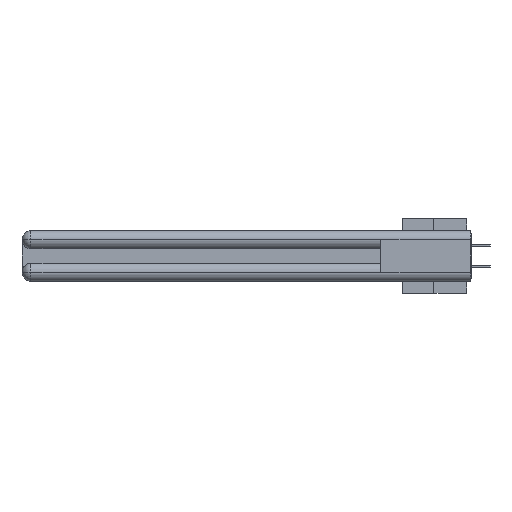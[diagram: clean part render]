
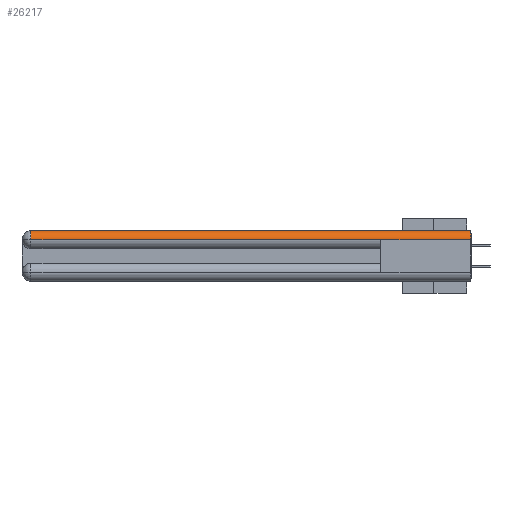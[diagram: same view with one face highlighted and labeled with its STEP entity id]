
A CAD part, left-side view. The second image highlights one B-rep face of the part: STEP entity #26217.
In plain terms, the highlighted cylindrical face has radius 1.562 mm (diameter 3.124 mm), a partial arc.
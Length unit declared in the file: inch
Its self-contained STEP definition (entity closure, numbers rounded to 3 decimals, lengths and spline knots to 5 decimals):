
#1424 = CARTESIAN_POINT ( 'NONE',  ( 0., 0., -0.0615 ) ) ;
#1854 = VERTEX_POINT ( 'NONE', #1424 ) ;
#3179 = VERTEX_POINT ( 'NONE', #27370 ) ;
#4358 = DIRECTION ( 'NONE',  ( 0., -1., 0. ) ) ;
#4647 = VECTOR ( 'NONE', #32517, 39.37008 ) ;
#5526 = ORIENTED_EDGE ( 'NONE', *, *, #14792, .F. ) ;
#6897 = VERTEX_POINT ( 'NONE', #30678 ) ;
#6945 = VERTEX_POINT ( 'NONE', #16879 ) ;
#8374 = EDGE_CURVE ( 'NONE', #6897, #30073, #10046, .T. ) ;
#8492 = EDGE_LOOP ( 'NONE', ( #33950, #23295, #24960, #5526, #19965 ) ) ;
#8724 = LINE ( 'NONE', #32281, #4647 ) ;
#10006 = CARTESIAN_POINT ( 'NONE',  ( 0., 3., -0.0615 ) ) ;
#10046 = CIRCLE ( 'NONE', #24034, 0.0615 ) ;
#11680 = DIRECTION ( 'NONE',  ( 0., 0., 1. ) ) ;
#11841 = VECTOR ( 'NONE', #4358, 39.37008 ) ;
#11908 = CARTESIAN_POINT ( 'NONE',  ( 0., 2.94, -0.0615 ) ) ;
#12241 = LINE ( 'NONE', #20618, #34445 ) ;
#13191 = CARTESIAN_POINT ( 'NONE',  ( 0.0615, 2.94, -0.0615 ) ) ;
#14202 = DIRECTION ( 'NONE',  ( 1., 0., 0. ) ) ;
#14792 = EDGE_CURVE ( 'NONE', #1854, #3179, #12241, .T. ) ;
#15182 = DIRECTION ( 'NONE',  ( 0., 1., 0. ) ) ;
#16879 = CARTESIAN_POINT ( 'NONE',  ( 0.0615, 0., 0. ) ) ;
#17101 = DIRECTION ( 'NONE',  ( 0., -1., 0. ) ) ;
#18936 = CARTESIAN_POINT ( 'NONE',  ( 0.0615, 0., -0.0615 ) ) ;
#19277 = AXIS2_PLACEMENT_3D ( 'NONE', #31559, #17101, #14202 ) ;
#19965 = ORIENTED_EDGE ( 'NONE', *, *, #31955, .F. ) ;
#20372 = LINE ( 'NONE', #10006, #11841 ) ;
#20618 = CARTESIAN_POINT ( 'NONE',  ( 0., 3., -0.0615 ) ) ;
#23295 = ORIENTED_EDGE ( 'NONE', *, *, #8374, .T. ) ;
#23879 = EDGE_CURVE ( 'NONE', #6897, #6945, #8724, .T. ) ;
#24034 = AXIS2_PLACEMENT_3D ( 'NONE', #13191, #36397, #36026 ) ;
#24771 = DIRECTION ( 'NONE',  ( 0., 1., 0. ) ) ;
#24960 = ORIENTED_EDGE ( 'NONE', *, *, #32616, .T. ) ;
#26056 = FACE_OUTER_BOUND ( 'NONE', #8492, .T. ) ;
#26217 = ADVANCED_FACE ( 'NONE', ( #26056 ), #32856, .T. ) ;
#27370 = CARTESIAN_POINT ( 'NONE',  ( 0., 0.6, -0.0615 ) ) ;
#30073 = VERTEX_POINT ( 'NONE', #11908 ) ;
#30678 = CARTESIAN_POINT ( 'NONE',  ( 0.0615, 2.94, 0. ) ) ;
#31274 = AXIS2_PLACEMENT_3D ( 'NONE', #18936, #24771, #11680 ) ;
#31559 = CARTESIAN_POINT ( 'NONE',  ( 0.0615, 0., -0.0615 ) ) ;
#31955 = EDGE_CURVE ( 'NONE', #6945, #1854, #36263, .T. ) ;
#32281 = CARTESIAN_POINT ( 'NONE',  ( 0.0615, 0., 0. ) ) ;
#32517 = DIRECTION ( 'NONE',  ( 0., -1., 0. ) ) ;
#32616 = EDGE_CURVE ( 'NONE', #30073, #3179, #20372, .T. ) ;
#32856 = CYLINDRICAL_SURFACE ( 'NONE', #31274, 0.0615 ) ;
#33950 = ORIENTED_EDGE ( 'NONE', *, *, #23879, .F. ) ;
#34445 = VECTOR ( 'NONE', #15182, 39.37008 ) ;
#36026 = DIRECTION ( 'NONE',  ( 0., 0., 1. ) ) ;
#36263 = CIRCLE ( 'NONE', #19277, 0.0615 ) ;
#36397 = DIRECTION ( 'NONE',  ( 0., -1., 0. ) ) ;
